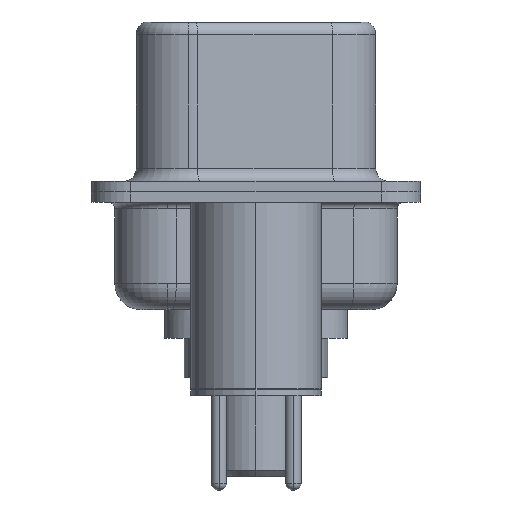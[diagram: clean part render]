
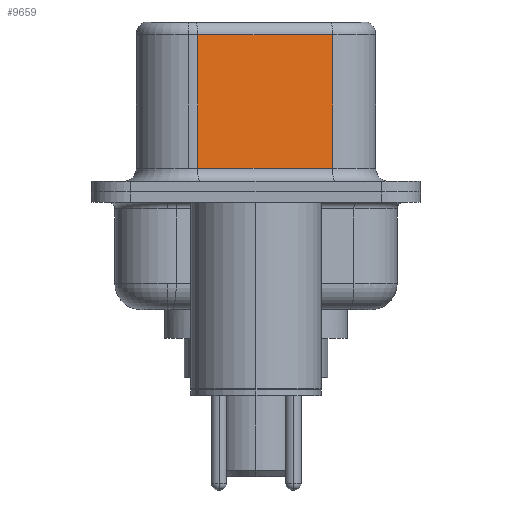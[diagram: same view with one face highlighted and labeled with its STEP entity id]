
A CAD part, left-side view. The second image highlights one B-rep face of the part: STEP entity #9659.
In plain terms, the highlighted planar face has unit normal (-0.985, -0.174, 0).
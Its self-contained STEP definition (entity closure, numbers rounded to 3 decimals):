
#586 = ORIENTED_EDGE ( 'NONE', *, *, #12935, .F. ) ;
#645 = ORIENTED_EDGE ( 'NONE', *, *, #13640, .T. ) ;
#1136 = DIRECTION ( 'NONE',  ( 0.985, 0.174, 0. ) ) ;
#1924 = ORIENTED_EDGE ( 'NONE', *, *, #5958, .T. ) ;
#3006 = LINE ( 'NONE', #5280, #6320 ) ;
#3190 = VECTOR ( 'NONE', #10513, 1000. ) ;
#3615 = LINE ( 'NONE', #16078, #3190 ) ;
#4063 = EDGE_CURVE ( 'NONE', #4578, #8442, #3006, .T. ) ;
#4578 = VERTEX_POINT ( 'NONE', #10394 ) ;
#5280 = CARTESIAN_POINT ( 'NONE',  ( 3.67, 2.233, 6.52 ) ) ;
#5690 = DIRECTION ( 'NONE',  ( 0.174, -0.985, 0. ) ) ;
#5958 = EDGE_CURVE ( 'NONE', #12882, #4578, #3615, .T. ) ;
#6320 = VECTOR ( 'NONE', #13382, 1000. ) ;
#7192 = VECTOR ( 'NONE', #5690, 1000. ) ;
#8098 = LINE ( 'NONE', #13760, #11406 ) ;
#8251 = VERTEX_POINT ( 'NONE', #13219 ) ;
#8442 = VERTEX_POINT ( 'NONE', #12063 ) ;
#9528 = CARTESIAN_POINT ( 'NONE',  ( 4.58, -2.927, 6.52 ) ) ;
#9599 = PLANE ( 'NONE',  #15858 ) ;
#9659 = ADVANCED_FACE ( 'NONE', ( #13426 ), #9599, .F. ) ;
#10394 = CARTESIAN_POINT ( 'NONE',  ( 3.67, 2.233, 6.02 ) ) ;
#10513 = DIRECTION ( 'NONE',  ( -0.174, 0.985, 0. ) ) ;
#11019 = DIRECTION ( 'NONE',  ( -0.174, 0.985, 0. ) ) ;
#11406 = VECTOR ( 'NONE', #15188, 1000. ) ;
#11492 = ORIENTED_EDGE ( 'NONE', *, *, #4063, .T. ) ;
#12063 = CARTESIAN_POINT ( 'NONE',  ( 3.67, 2.233, 0.9 ) ) ;
#12709 = CARTESIAN_POINT ( 'NONE',  ( 4.58, -2.927, 0.9 ) ) ;
#12882 = VERTEX_POINT ( 'NONE', #16461 ) ;
#12935 = EDGE_CURVE ( 'NONE', #12882, #8251, #8098, .T. ) ;
#13078 = EDGE_LOOP ( 'NONE', ( #586, #1924, #11492, #645 ) ) ;
#13219 = CARTESIAN_POINT ( 'NONE',  ( 4.58, -2.927, 0.9 ) ) ;
#13382 = DIRECTION ( 'NONE',  ( 0., 0., -1. ) ) ;
#13426 = FACE_OUTER_BOUND ( 'NONE', #13078, .T. ) ;
#13640 = EDGE_CURVE ( 'NONE', #8442, #8251, #15118, .T. ) ;
#13760 = CARTESIAN_POINT ( 'NONE',  ( 4.58, -2.927, 6.52 ) ) ;
#15118 = LINE ( 'NONE', #12709, #7192 ) ;
#15188 = DIRECTION ( 'NONE',  ( 0., 0., -1. ) ) ;
#15858 = AXIS2_PLACEMENT_3D ( 'NONE', #9528, #1136, #11019 ) ;
#16078 = CARTESIAN_POINT ( 'NONE',  ( 4.58, -2.927, 6.02 ) ) ;
#16461 = CARTESIAN_POINT ( 'NONE',  ( 4.58, -2.927, 6.02 ) ) ;
